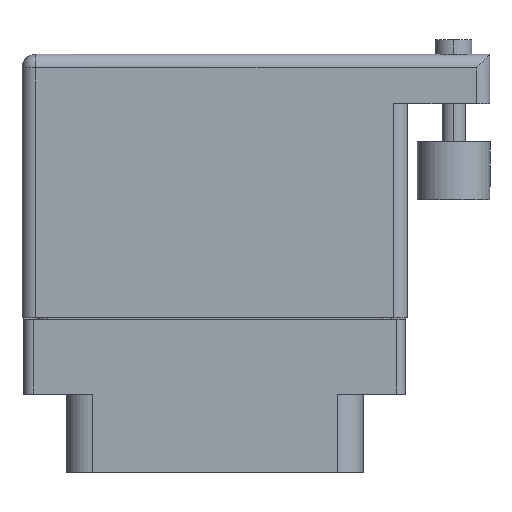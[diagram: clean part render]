
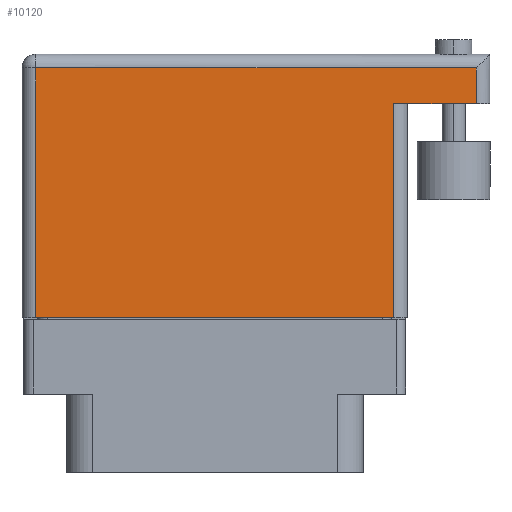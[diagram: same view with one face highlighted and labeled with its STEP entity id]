
A CAD part, front view. The second image highlights one B-rep face of the part: STEP entity #10120.
In plain terms, the highlighted face is planar.
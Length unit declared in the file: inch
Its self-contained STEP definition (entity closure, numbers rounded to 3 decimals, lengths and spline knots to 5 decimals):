
#522 = DIRECTION ( 'NONE',  ( 1., 0., 0. ) ) ;
#843 = LINE ( 'NONE', #8020, #14666 ) ;
#2050 = CARTESIAN_POINT ( 'NONE',  ( 0.6155, 0.636, 0.3575 ) ) ;
#2102 = CARTESIAN_POINT ( 'NONE',  ( 0.6155, 0.636, 0.3575 ) ) ;
#2400 = LINE ( 'NONE', #23129, #13704 ) ;
#2911 = DIRECTION ( 'NONE',  ( 0., -1., 0. ) ) ;
#3503 = CARTESIAN_POINT ( 'NONE',  ( -0.6625, 0.806, 0.3575 ) ) ;
#3651 = ORIENTED_EDGE ( 'NONE', *, *, #24738, .T. ) ;
#4180 = VECTOR ( 'NONE', #2911, 39.37008 ) ;
#4839 = VERTEX_POINT ( 'NONE', #10518 ) ;
#6380 = EDGE_CURVE ( 'NONE', #27816, #4839, #17696, .T. ) ;
#6866 = CARTESIAN_POINT ( 'NONE',  ( 0.6155, -0.1, 0.3575 ) ) ;
#7760 = DIRECTION ( 'NONE',  ( 0., 1., 0. ) ) ;
#7887 = EDGE_CURVE ( 'NONE', #24118, #12334, #23874, .T. ) ;
#7915 = CARTESIAN_POINT ( 'NONE',  ( 0.8995, 0.806, 0.3575 ) ) ;
#8020 = CARTESIAN_POINT ( 'NONE',  ( -0.6625, -0.1, 0.3575 ) ) ;
#8046 = DIRECTION ( 'NONE',  ( 0., 0., -1. ) ) ;
#8414 = VECTOR ( 'NONE', #10678, 39.37008 ) ;
#9393 = CARTESIAN_POINT ( 'NONE',  ( 0.8995, 0.759, 0.3575 ) ) ;
#9987 = EDGE_LOOP ( 'NONE', ( #11535, #23427, #30535, #19197, #20955, #3651 ) ) ;
#10120 = ADVANCED_FACE ( 'NONE', ( #22376 ), #20361, .F. ) ;
#10518 = CARTESIAN_POINT ( 'NONE',  ( -0.6155, 0.759, 0.3575 ) ) ;
#10525 = CARTESIAN_POINT ( 'NONE',  ( -0.6625, 0.759, 0.3575 ) ) ;
#10678 = DIRECTION ( 'NONE',  ( -1., 0., 0. ) ) ;
#10691 = VECTOR ( 'NONE', #7760, 39.37008 ) ;
#11006 = DIRECTION ( 'NONE',  ( -1., 0., 0. ) ) ;
#11535 = ORIENTED_EDGE ( 'NONE', *, *, #29439, .T. ) ;
#11959 = VERTEX_POINT ( 'NONE', #14396 ) ;
#12334 = VERTEX_POINT ( 'NONE', #2102 ) ;
#12866 = EDGE_CURVE ( 'NONE', #11959, #12334, #2400, .T. ) ;
#13488 = VECTOR ( 'NONE', #23262, 39.37008 ) ;
#13704 = VECTOR ( 'NONE', #19082, 39.37008 ) ;
#14396 = CARTESIAN_POINT ( 'NONE',  ( 0.8995, 0.636, 0.3575 ) ) ;
#14666 = VECTOR ( 'NONE', #522, 39.37008 ) ;
#17696 = LINE ( 'NONE', #10525, #8414 ) ;
#19082 = DIRECTION ( 'NONE',  ( -1., 0., 0. ) ) ;
#19197 = ORIENTED_EDGE ( 'NONE', *, *, #24632, .T. ) ;
#19597 = CARTESIAN_POINT ( 'NONE',  ( -0.6155, -0.1, 0.3575 ) ) ;
#20361 = PLANE ( 'NONE',  #26185 ) ;
#20955 = ORIENTED_EDGE ( 'NONE', *, *, #6380, .T. ) ;
#21600 = CARTESIAN_POINT ( 'NONE',  ( -0.6155, -0.1, 0.3575 ) ) ;
#22376 = FACE_OUTER_BOUND ( 'NONE', #9987, .T. ) ;
#23129 = CARTESIAN_POINT ( 'NONE',  ( 0.9465, 0.636, 0.3575 ) ) ;
#23231 = VERTEX_POINT ( 'NONE', #21600 ) ;
#23262 = DIRECTION ( 'NONE',  ( 0., 1., 0. ) ) ;
#23427 = ORIENTED_EDGE ( 'NONE', *, *, #7887, .T. ) ;
#23874 = LINE ( 'NONE', #2050, #13488 ) ;
#23936 = LINE ( 'NONE', #7915, #10691 ) ;
#24118 = VERTEX_POINT ( 'NONE', #6866 ) ;
#24257 = LINE ( 'NONE', #19597, #4180 ) ;
#24632 = EDGE_CURVE ( 'NONE', #11959, #27816, #23936, .T. ) ;
#24738 = EDGE_CURVE ( 'NONE', #4839, #23231, #24257, .T. ) ;
#26185 = AXIS2_PLACEMENT_3D ( 'NONE', #3503, #8046, #11006 ) ;
#27816 = VERTEX_POINT ( 'NONE', #9393 ) ;
#29439 = EDGE_CURVE ( 'NONE', #23231, #24118, #843, .T. ) ;
#30535 = ORIENTED_EDGE ( 'NONE', *, *, #12866, .F. ) ;
